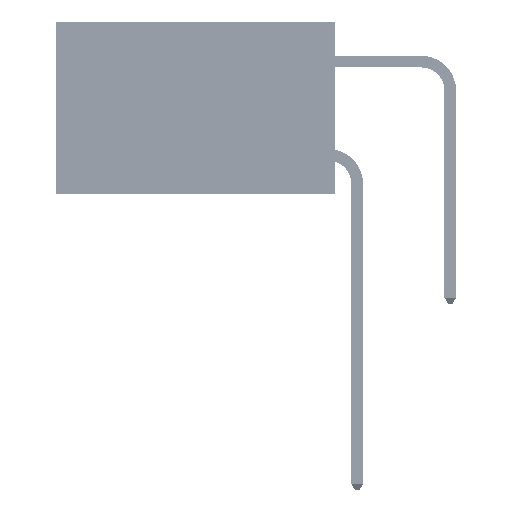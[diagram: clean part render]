
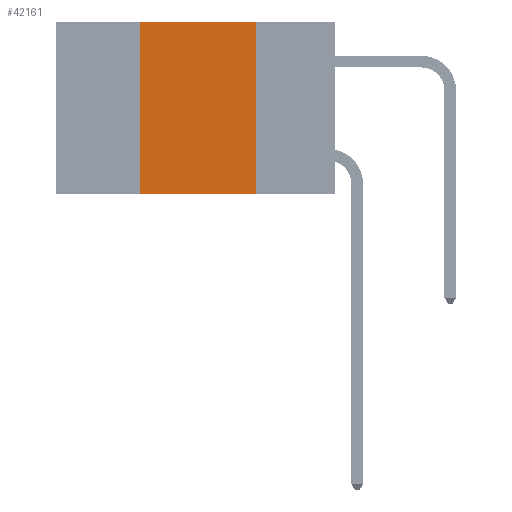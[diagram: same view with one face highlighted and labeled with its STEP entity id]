
A CAD part, left-side view. The second image highlights one B-rep face of the part: STEP entity #42161.
In plain terms, the highlighted planar face has unit normal (-1, 0, 0).
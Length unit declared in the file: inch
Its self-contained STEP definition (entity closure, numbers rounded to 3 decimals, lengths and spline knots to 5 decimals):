
#765 = LINE ( 'NONE', #47499, #11212 ) ;
#3255 = VERTEX_POINT ( 'NONE', #38438 ) ;
#3753 = LINE ( 'NONE', #10641, #39370 ) ;
#3778 = DIRECTION ( 'NONE',  ( 0., 0., -1. ) ) ;
#5422 = CARTESIAN_POINT ( 'NONE',  ( 0., 0.17, 0. ) ) ;
#6850 = EDGE_CURVE ( 'NONE', #3255, #33660, #24537, .T. ) ;
#7838 = EDGE_CURVE ( 'NONE', #15651, #32374, #3753, .T. ) ;
#8626 = ORIENTED_EDGE ( 'NONE', *, *, #7838, .F. ) ;
#8942 = AXIS2_PLACEMENT_3D ( 'NONE', #43643, #15638, #3778 ) ;
#10641 = CARTESIAN_POINT ( 'NONE',  ( 0., 0.42, 0. ) ) ;
#11038 = EDGE_CURVE ( 'NONE', #15651, #33660, #765, .T. ) ;
#11212 = VECTOR ( 'NONE', #26617, 39.37008 ) ;
#13664 = VECTOR ( 'NONE', #42683, 39.37008 ) ;
#14567 = DIRECTION ( 'NONE',  ( 0., -1., 0. ) ) ;
#14991 = DIRECTION ( 'NONE',  ( 0., 0., 1. ) ) ;
#15638 = DIRECTION ( 'NONE',  ( 1., 0., 0. ) ) ;
#15651 = VERTEX_POINT ( 'NONE', #34006 ) ;
#20491 = CARTESIAN_POINT ( 'NONE',  ( 0., 0.17, -0.37 ) ) ;
#22177 = CARTESIAN_POINT ( 'NONE',  ( 0., 0.42, 0. ) ) ;
#22460 = CARTESIAN_POINT ( 'NONE',  ( 0., 0.6, 0. ) ) ;
#24537 = LINE ( 'NONE', #5422, #13664 ) ;
#26617 = DIRECTION ( 'NONE',  ( 0., -1., 0. ) ) ;
#32374 = VERTEX_POINT ( 'NONE', #22177 ) ;
#33660 = VERTEX_POINT ( 'NONE', #20491 ) ;
#34006 = CARTESIAN_POINT ( 'NONE',  ( 0., 0.42, -0.37 ) ) ;
#35801 = EDGE_CURVE ( 'NONE', #32374, #3255, #43947, .T. ) ;
#35993 = PLANE ( 'NONE',  #8942 ) ;
#38438 = CARTESIAN_POINT ( 'NONE',  ( 0., 0.17, 0. ) ) ;
#39309 = FACE_OUTER_BOUND ( 'NONE', #51860, .T. ) ;
#39370 = VECTOR ( 'NONE', #14991, 39.37008 ) ;
#41668 = ORIENTED_EDGE ( 'NONE', *, *, #11038, .T. ) ;
#42161 = ADVANCED_FACE ( 'NONE', ( #39309 ), #35993, .F. ) ;
#42683 = DIRECTION ( 'NONE',  ( 0., 0., -1. ) ) ;
#43643 = CARTESIAN_POINT ( 'NONE',  ( 0., 0.6, 0. ) ) ;
#43947 = LINE ( 'NONE', #22460, #47176 ) ;
#46492 = ORIENTED_EDGE ( 'NONE', *, *, #6850, .F. ) ;
#47176 = VECTOR ( 'NONE', #14567, 39.37008 ) ;
#47499 = CARTESIAN_POINT ( 'NONE',  ( 0., 0.6, -0.37 ) ) ;
#49960 = ORIENTED_EDGE ( 'NONE', *, *, #35801, .F. ) ;
#51860 = EDGE_LOOP ( 'NONE', ( #46492, #49960, #8626, #41668 ) ) ;
